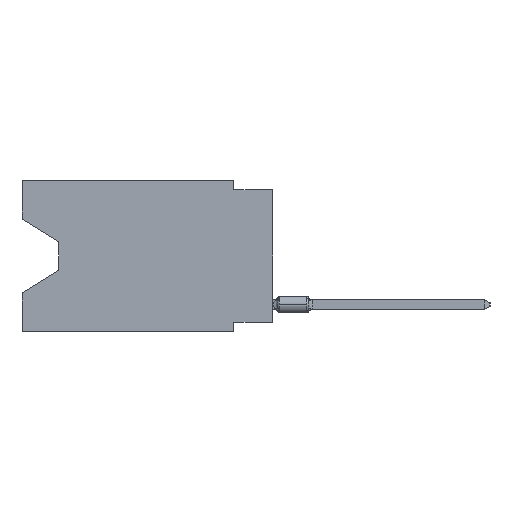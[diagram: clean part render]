
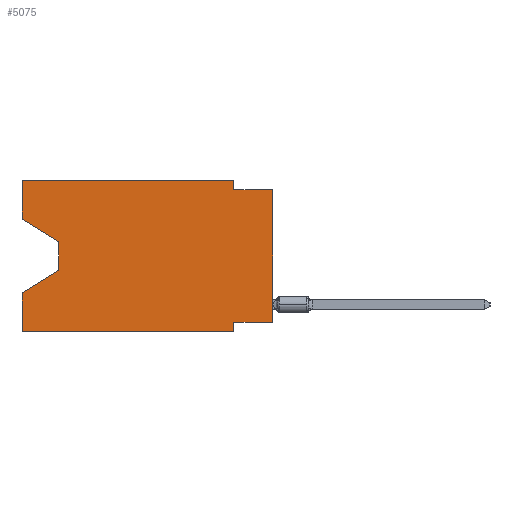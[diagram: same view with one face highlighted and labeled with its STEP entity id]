
A CAD part, left-side view. The second image highlights one B-rep face of the part: STEP entity #5075.
In plain terms, the highlighted planar face has unit normal (-1, 0, 0).
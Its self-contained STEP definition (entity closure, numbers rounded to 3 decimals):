
#438 = ORIENTED_EDGE ( 'NONE', *, *, #33396, .T. ) ;
#721 = VECTOR ( 'NONE', #35654, 1000. ) ;
#1441 = DIRECTION ( 'NONE',  ( 0., -1., 0. ) ) ;
#1912 = CARTESIAN_POINT ( 'NONE',  ( 0., 0., -0.635 ) ) ;
#2055 = ORIENTED_EDGE ( 'NONE', *, *, #33983, .T. ) ;
#2072 = VERTEX_POINT ( 'NONE', #11097 ) ;
#3427 = DIRECTION ( 'NONE',  ( 0., 0., 1. ) ) ;
#3710 = FACE_OUTER_BOUND ( 'NONE', #16753, .T. ) ;
#4178 = CARTESIAN_POINT ( 'NONE',  ( 0., 16.383, -9.906 ) ) ;
#4374 = CARTESIAN_POINT ( 'NONE',  ( 0., 16.383, -2.546 ) ) ;
#4709 = LINE ( 'NONE', #18760, #8068 ) ;
#4798 = VECTOR ( 'NONE', #3427, 1000. ) ;
#5001 = CARTESIAN_POINT ( 'NONE',  ( 0., 2.54, 0. ) ) ;
#5010 = CARTESIAN_POINT ( 'NONE',  ( 0., 16.383, 0. ) ) ;
#5075 = ADVANCED_FACE ( 'NONE', ( #3710 ), #14854, .F. ) ;
#5938 = LINE ( 'NONE', #31301, #25308 ) ;
#6065 = ORIENTED_EDGE ( 'NONE', *, *, #25204, .F. ) ;
#6164 = LINE ( 'NONE', #17286, #4798 ) ;
#6435 = CARTESIAN_POINT ( 'NONE',  ( 0., 16.383, 0. ) ) ;
#6601 = VERTEX_POINT ( 'NONE', #11319 ) ;
#6877 = DIRECTION ( 'NONE',  ( 0., 0., 1. ) ) ;
#6878 = VERTEX_POINT ( 'NONE', #28806 ) ;
#7851 = LINE ( 'NONE', #4374, #11350 ) ;
#7950 = LINE ( 'NONE', #1912, #31764 ) ;
#8068 = VECTOR ( 'NONE', #26993, 1000. ) ;
#8224 = VERTEX_POINT ( 'NONE', #24098 ) ;
#9501 = VECTOR ( 'NONE', #16137, 1000. ) ;
#11097 = CARTESIAN_POINT ( 'NONE',  ( 0., 2.54, 0. ) ) ;
#11319 = CARTESIAN_POINT ( 'NONE',  ( 0., 13.97, -4.013 ) ) ;
#11350 = VECTOR ( 'NONE', #32112, 1000. ) ;
#12113 = VECTOR ( 'NONE', #1441, 1000. ) ;
#12402 = CARTESIAN_POINT ( 'NONE',  ( 0., 2.54, -9.906 ) ) ;
#12584 = LINE ( 'NONE', #4178, #12113 ) ;
#12821 = DIRECTION ( 'NONE',  ( 1., 0., 0. ) ) ;
#12907 = EDGE_CURVE ( 'NONE', #6878, #13426, #6164, .T. ) ;
#13180 = LINE ( 'NONE', #26871, #35221 ) ;
#13231 = EDGE_CURVE ( 'NONE', #13426, #2072, #32570, .T. ) ;
#13258 = VERTEX_POINT ( 'NONE', #18495 ) ;
#13426 = VERTEX_POINT ( 'NONE', #6435 ) ;
#13599 = EDGE_CURVE ( 'NONE', #31647, #35620, #13180, .T. ) ;
#13991 = EDGE_CURVE ( 'NONE', #6878, #6601, #7851, .T. ) ;
#14854 = PLANE ( 'NONE',  #26356 ) ;
#14935 = VERTEX_POINT ( 'NONE', #32799 ) ;
#15606 = DIRECTION ( 'NONE',  ( 0., -1., 0. ) ) ;
#16137 = DIRECTION ( 'NONE',  ( 0., -1., 0. ) ) ;
#16753 = EDGE_LOOP ( 'NONE', ( #19711, #438, #29583, #31612, #2055, #36041, #29323, #35648, #33442, #6065, #32311, #22921 ) ) ;
#17277 = CARTESIAN_POINT ( 'NONE',  ( 0., 16.383, 0. ) ) ;
#17286 = CARTESIAN_POINT ( 'NONE',  ( 0., 16.383, 0. ) ) ;
#17411 = DIRECTION ( 'NONE',  ( 0., 0., 1. ) ) ;
#17924 = CARTESIAN_POINT ( 'NONE',  ( 0., 16.383, 0. ) ) ;
#18495 = CARTESIAN_POINT ( 'NONE',  ( 0., 0., -0.635 ) ) ;
#18760 = CARTESIAN_POINT ( 'NONE',  ( 0., 2.54, -9.906 ) ) ;
#19078 = CARTESIAN_POINT ( 'NONE',  ( 0., 13.97, -4.013 ) ) ;
#19711 = ORIENTED_EDGE ( 'NONE', *, *, #13991, .T. ) ;
#20734 = CARTESIAN_POINT ( 'NONE',  ( 0., 13.97, -5.893 ) ) ;
#21619 = CARTESIAN_POINT ( 'NONE',  ( 0., 16.383, -9.906 ) ) ;
#22147 = EDGE_CURVE ( 'NONE', #31647, #13258, #5938, .T. ) ;
#22345 = VECTOR ( 'NONE', #6877, 1000. ) ;
#22921 = ORIENTED_EDGE ( 'NONE', *, *, #12907, .F. ) ;
#23435 = VERTEX_POINT ( 'NONE', #12402 ) ;
#23821 = EDGE_CURVE ( 'NONE', #27817, #25708, #31526, .T. ) ;
#24098 = CARTESIAN_POINT ( 'NONE',  ( 0., 2.54, -0.635 ) ) ;
#24709 = LINE ( 'NONE', #5001, #721 ) ;
#25104 = CARTESIAN_POINT ( 'NONE',  ( 0., 0., -9.271 ) ) ;
#25113 = LINE ( 'NONE', #19078, #28959 ) ;
#25204 = EDGE_CURVE ( 'NONE', #2072, #8224, #24709, .T. ) ;
#25308 = VECTOR ( 'NONE', #17411, 1000. ) ;
#25708 = VERTEX_POINT ( 'NONE', #30979 ) ;
#25860 = EDGE_CURVE ( 'NONE', #14935, #25708, #29681, .T. ) ;
#25990 = DIRECTION ( 'NONE',  ( 0., 0., -1. ) ) ;
#26356 = AXIS2_PLACEMENT_3D ( 'NONE', #17924, #12821, #25990 ) ;
#26871 = CARTESIAN_POINT ( 'NONE',  ( 0., 0., -9.271 ) ) ;
#26993 = DIRECTION ( 'NONE',  ( 0., 0., -1. ) ) ;
#27817 = VERTEX_POINT ( 'NONE', #21619 ) ;
#27822 = EDGE_CURVE ( 'NONE', #8224, #13258, #7950, .T. ) ;
#28806 = CARTESIAN_POINT ( 'NONE',  ( 0., 16.383, -2.546 ) ) ;
#28959 = VECTOR ( 'NONE', #35885, 1000. ) ;
#29295 = CARTESIAN_POINT ( 'NONE',  ( 0., 2.54, -9.271 ) ) ;
#29323 = ORIENTED_EDGE ( 'NONE', *, *, #13599, .F. ) ;
#29327 = DIRECTION ( 'NONE',  ( 0., 0.855, -0.519 ) ) ;
#29425 = DIRECTION ( 'NONE',  ( 0., 1., 0. ) ) ;
#29583 = ORIENTED_EDGE ( 'NONE', *, *, #25860, .T. ) ;
#29681 = LINE ( 'NONE', #20734, #31060 ) ;
#30979 = CARTESIAN_POINT ( 'NONE',  ( 0., 16.383, -7.36 ) ) ;
#31060 = VECTOR ( 'NONE', #29327, 1000. ) ;
#31301 = CARTESIAN_POINT ( 'NONE',  ( 0., 0., 0. ) ) ;
#31526 = LINE ( 'NONE', #17277, #22345 ) ;
#31612 = ORIENTED_EDGE ( 'NONE', *, *, #23821, .F. ) ;
#31647 = VERTEX_POINT ( 'NONE', #25104 ) ;
#31764 = VECTOR ( 'NONE', #15606, 1000. ) ;
#32112 = DIRECTION ( 'NONE',  ( 0., -0.855, -0.519 ) ) ;
#32311 = ORIENTED_EDGE ( 'NONE', *, *, #13231, .F. ) ;
#32570 = LINE ( 'NONE', #5010, #9501 ) ;
#32799 = CARTESIAN_POINT ( 'NONE',  ( 0., 13.97, -5.893 ) ) ;
#32995 = EDGE_CURVE ( 'NONE', #35620, #23435, #4709, .T. ) ;
#33396 = EDGE_CURVE ( 'NONE', #6601, #14935, #25113, .T. ) ;
#33442 = ORIENTED_EDGE ( 'NONE', *, *, #27822, .F. ) ;
#33983 = EDGE_CURVE ( 'NONE', #27817, #23435, #12584, .T. ) ;
#35221 = VECTOR ( 'NONE', #29425, 1000. ) ;
#35620 = VERTEX_POINT ( 'NONE', #29295 ) ;
#35648 = ORIENTED_EDGE ( 'NONE', *, *, #22147, .T. ) ;
#35654 = DIRECTION ( 'NONE',  ( 0., 0., -1. ) ) ;
#35885 = DIRECTION ( 'NONE',  ( 0., 0., -1. ) ) ;
#36041 = ORIENTED_EDGE ( 'NONE', *, *, #32995, .F. ) ;
